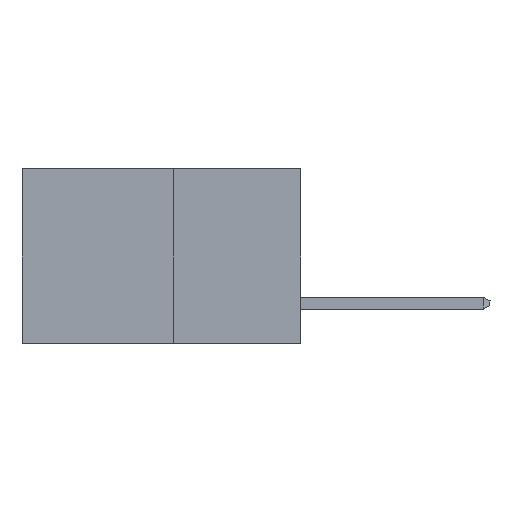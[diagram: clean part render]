
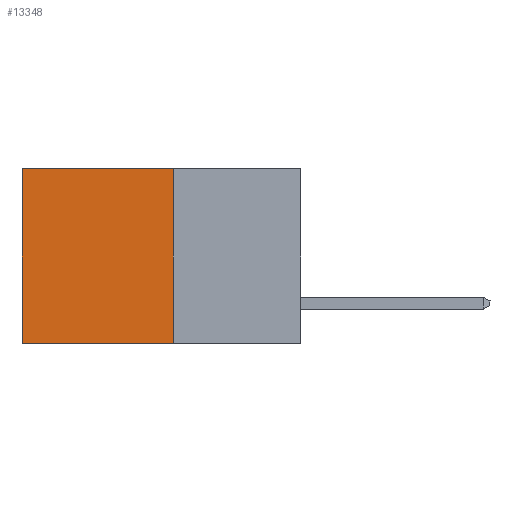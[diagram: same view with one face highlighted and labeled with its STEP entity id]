
A CAD part, left-side view. The second image highlights one B-rep face of the part: STEP entity #13348.
In plain terms, the highlighted planar face has unit normal (-1, 0, 0).
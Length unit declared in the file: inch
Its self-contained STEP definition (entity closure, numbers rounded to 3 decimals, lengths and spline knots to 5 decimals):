
#33 = CARTESIAN_POINT ( 'NONE',  ( 0.277, 0.59, -0.37 ) ) ;
#156 = EDGE_LOOP ( 'NONE', ( #787, #10578, #2737, #5318 ) ) ;
#420 = VECTOR ( 'NONE', #14032, 39.37008 ) ;
#787 = ORIENTED_EDGE ( 'NONE', *, *, #5247, .T. ) ;
#1661 = CARTESIAN_POINT ( 'NONE',  ( 0.277, 0.27, 0. ) ) ;
#2046 = CARTESIAN_POINT ( 'NONE',  ( 0.277, 0.59, 0. ) ) ;
#2704 = EDGE_CURVE ( 'NONE', #12384, #13065, #5794, .T. ) ;
#2737 = ORIENTED_EDGE ( 'NONE', *, *, #4579, .F. ) ;
#3296 = CARTESIAN_POINT ( 'NONE',  ( 0.277, 0.27, -0.37 ) ) ;
#4282 = CARTESIAN_POINT ( 'NONE',  ( 0.277, 0.27, -0.37 ) ) ;
#4468 = DIRECTION ( 'NONE',  ( 1., 0., 0. ) ) ;
#4579 = EDGE_CURVE ( 'NONE', #14490, #12384, #6075, .T. ) ;
#5247 = EDGE_CURVE ( 'NONE', #11750, #13065, #12465, .T. ) ;
#5318 = ORIENTED_EDGE ( 'NONE', *, *, #11146, .T. ) ;
#5794 = LINE ( 'NONE', #8679, #11550 ) ;
#6075 = LINE ( 'NONE', #7542, #11794 ) ;
#6185 = FACE_OUTER_BOUND ( 'NONE', #156, .T. ) ;
#7542 = CARTESIAN_POINT ( 'NONE',  ( 0.277, 0.27, -0.37 ) ) ;
#7563 = DIRECTION ( 'NONE',  ( 0., 0., -1. ) ) ;
#7722 = CARTESIAN_POINT ( 'NONE',  ( 0.277, 0.59, -0.37 ) ) ;
#7846 = CARTESIAN_POINT ( 'NONE',  ( 0.277, 0.27, 0. ) ) ;
#8679 = CARTESIAN_POINT ( 'NONE',  ( 0.277, 0.27, -0.37 ) ) ;
#10148 = AXIS2_PLACEMENT_3D ( 'NONE', #3296, #4468, #12471 ) ;
#10268 = PLANE ( 'NONE',  #10148 ) ;
#10289 = DIRECTION ( 'NONE',  ( 0., 1., 0. ) ) ;
#10578 = ORIENTED_EDGE ( 'NONE', *, *, #2704, .F. ) ;
#10921 = VECTOR ( 'NONE', #14377, 39.37008 ) ;
#11146 = EDGE_CURVE ( 'NONE', #14490, #11750, #14062, .T. ) ;
#11550 = VECTOR ( 'NONE', #10289, 39.37008 ) ;
#11750 = VERTEX_POINT ( 'NONE', #2046 ) ;
#11794 = VECTOR ( 'NONE', #7563, 39.37008 ) ;
#12384 = VERTEX_POINT ( 'NONE', #4282 ) ;
#12465 = LINE ( 'NONE', #33, #420 ) ;
#12471 = DIRECTION ( 'NONE',  ( 0., 0., -1. ) ) ;
#13065 = VERTEX_POINT ( 'NONE', #7722 ) ;
#13348 = ADVANCED_FACE ( 'NONE', ( #6185 ), #10268, .F. ) ;
#14032 = DIRECTION ( 'NONE',  ( 0., 0., -1. ) ) ;
#14062 = LINE ( 'NONE', #7846, #10921 ) ;
#14377 = DIRECTION ( 'NONE',  ( 0., 1., 0. ) ) ;
#14490 = VERTEX_POINT ( 'NONE', #1661 ) ;
